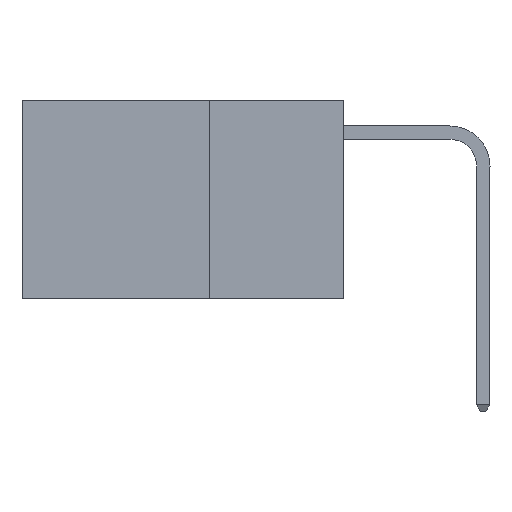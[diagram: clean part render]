
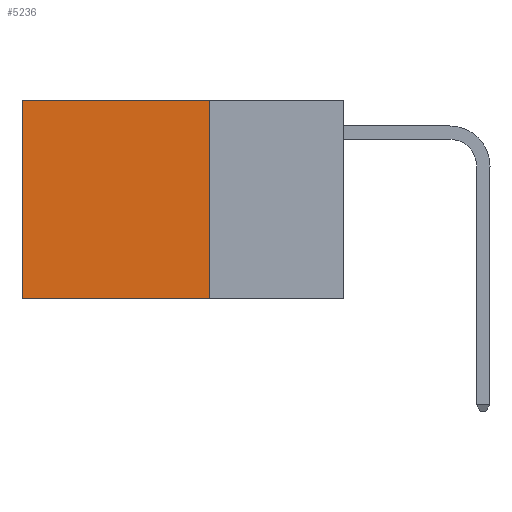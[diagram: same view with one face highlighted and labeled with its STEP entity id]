
A CAD part, left-side view. The second image highlights one B-rep face of the part: STEP entity #5236.
In plain terms, the highlighted planar face has unit normal (-1, 0, 0).
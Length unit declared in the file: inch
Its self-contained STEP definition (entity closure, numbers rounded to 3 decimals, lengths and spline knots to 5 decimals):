
#116 = LINE ( 'NONE', #15342, #10006 ) ;
#334 = DIRECTION ( 'NONE',  ( 0., 0., -1. ) ) ;
#1121 = VECTOR ( 'NONE', #5564, 39.37008 ) ;
#1771 = EDGE_CURVE ( 'NONE', #16356, #2358, #6260, .T. ) ;
#1949 = CARTESIAN_POINT ( 'NONE',  ( 0.2625, 0.25, 0. ) ) ;
#1984 = DIRECTION ( 'NONE',  ( 0., 0., -1. ) ) ;
#2358 = VERTEX_POINT ( 'NONE', #4380 ) ;
#2395 = EDGE_LOOP ( 'NONE', ( #5878, #14017, #13496, #7481 ) ) ;
#2426 = CARTESIAN_POINT ( 'NONE',  ( 0.2625, 0.6, 0. ) ) ;
#3513 = EDGE_CURVE ( 'NONE', #2358, #8664, #116, .T. ) ;
#4380 = CARTESIAN_POINT ( 'NONE',  ( 0.2625, 0.25, -0.37 ) ) ;
#4679 = CARTESIAN_POINT ( 'NONE',  ( 0.2625, 0.25, 0. ) ) ;
#5236 = ADVANCED_FACE ( 'NONE', ( #7714 ), #7159, .F. ) ;
#5564 = DIRECTION ( 'NONE',  ( 0., 0., -1. ) ) ;
#5871 = CARTESIAN_POINT ( 'NONE',  ( 0.2625, 0.25, 0. ) ) ;
#5878 = ORIENTED_EDGE ( 'NONE', *, *, #14713, .T. ) ;
#6260 = LINE ( 'NONE', #1949, #12247 ) ;
#6850 = VECTOR ( 'NONE', #12320, 39.37008 ) ;
#7159 = PLANE ( 'NONE',  #13733 ) ;
#7481 = ORIENTED_EDGE ( 'NONE', *, *, #16567, .T. ) ;
#7714 = FACE_OUTER_BOUND ( 'NONE', #2395, .T. ) ;
#8487 = DIRECTION ( 'NONE',  ( 1., 0., 0. ) ) ;
#8664 = VERTEX_POINT ( 'NONE', #10745 ) ;
#10006 = VECTOR ( 'NONE', #11643, 39.37008 ) ;
#10565 = VERTEX_POINT ( 'NONE', #2426 ) ;
#10650 = LINE ( 'NONE', #4679, #6850 ) ;
#10745 = CARTESIAN_POINT ( 'NONE',  ( 0.2625, 0.6, -0.37 ) ) ;
#11643 = DIRECTION ( 'NONE',  ( 0., 1., 0. ) ) ;
#11933 = CARTESIAN_POINT ( 'NONE',  ( 0.2625, 0.6, 0. ) ) ;
#12247 = VECTOR ( 'NONE', #1984, 39.37008 ) ;
#12320 = DIRECTION ( 'NONE',  ( 0., 1., 0. ) ) ;
#13496 = ORIENTED_EDGE ( 'NONE', *, *, #1771, .F. ) ;
#13733 = AXIS2_PLACEMENT_3D ( 'NONE', #5871, #8487, #334 ) ;
#14017 = ORIENTED_EDGE ( 'NONE', *, *, #3513, .F. ) ;
#14713 = EDGE_CURVE ( 'NONE', #10565, #8664, #15370, .T. ) ;
#15342 = CARTESIAN_POINT ( 'NONE',  ( 0.2625, 0.25, -0.37 ) ) ;
#15370 = LINE ( 'NONE', #11933, #1121 ) ;
#15760 = CARTESIAN_POINT ( 'NONE',  ( 0.2625, 0.25, 0. ) ) ;
#16356 = VERTEX_POINT ( 'NONE', #15760 ) ;
#16567 = EDGE_CURVE ( 'NONE', #16356, #10565, #10650, .T. ) ;
